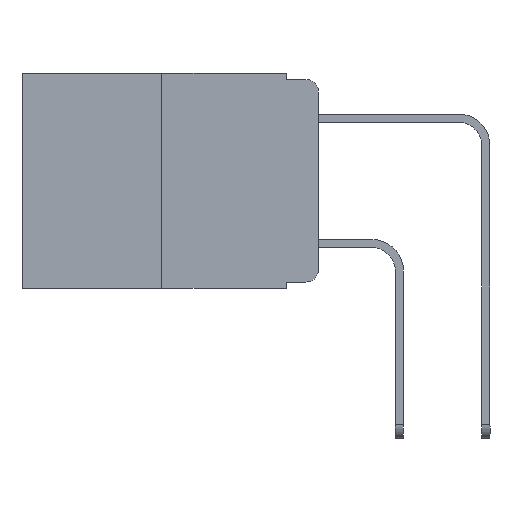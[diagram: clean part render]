
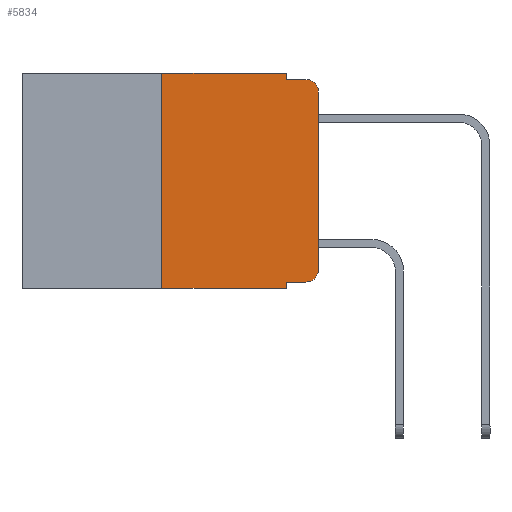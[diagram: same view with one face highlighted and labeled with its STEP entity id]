
A CAD part, left-side view. The second image highlights one B-rep face of the part: STEP entity #5834.
In plain terms, the highlighted planar face has unit normal (-1, 0, 0).
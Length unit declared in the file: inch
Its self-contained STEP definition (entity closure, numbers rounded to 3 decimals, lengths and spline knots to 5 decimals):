
#382 = CARTESIAN_POINT ( 'NONE',  ( 0., 0.051, -0.333 ) ) ;
#771 = CARTESIAN_POINT ( 'NONE',  ( 0., 0.25, 0. ) ) ;
#827 = CARTESIAN_POINT ( 'NONE',  ( 0., 0.473, 0. ) ) ;
#883 = CARTESIAN_POINT ( 'NONE',  ( 0., 0., 0. ) ) ;
#1315 = EDGE_CURVE ( 'NONE', #7490, #17654, #11008, .T. ) ;
#1879 = CARTESIAN_POINT ( 'NONE',  ( 0., 0.051, -0.343 ) ) ;
#2138 = DIRECTION ( 'NONE',  ( 0., 0., 1. ) ) ;
#2146 = DIRECTION ( 'NONE',  ( -1., 0., 0. ) ) ;
#2339 = CARTESIAN_POINT ( 'NONE',  ( 0., 0.051, 0. ) ) ;
#2368 = DIRECTION ( 'NONE',  ( -1., 0., 0. ) ) ;
#2535 = DIRECTION ( 'NONE',  ( 0., -1., 0. ) ) ;
#2853 = EDGE_CURVE ( 'NONE', #7490, #3936, #18631, .T. ) ;
#3482 = EDGE_CURVE ( 'NONE', #6286, #12022, #12248, .T. ) ;
#3511 = ORIENTED_EDGE ( 'NONE', *, *, #8426, .F. ) ;
#3579 = ORIENTED_EDGE ( 'NONE', *, *, #7062, .F. ) ;
#3762 = LINE ( 'NONE', #17247, #12461 ) ;
#3936 = VERTEX_POINT ( 'NONE', #6505 ) ;
#3972 = ORIENTED_EDGE ( 'NONE', *, *, #3482, .T. ) ;
#4372 = AXIS2_PLACEMENT_3D ( 'NONE', #827, #8157, #5220 ) ;
#4924 = EDGE_CURVE ( 'NONE', #9621, #9462, #5267, .T. ) ;
#5220 = DIRECTION ( 'NONE',  ( 0., 0., -1. ) ) ;
#5251 = DIRECTION ( 'NONE',  ( 0., 0., -1. ) ) ;
#5267 = LINE ( 'NONE', #5469, #11663 ) ;
#5469 = CARTESIAN_POINT ( 'NONE',  ( 0., 0.051, -0.01 ) ) ;
#5834 = ADVANCED_FACE ( 'NONE', ( #9622 ), #12666, .F. ) ;
#5928 = VECTOR ( 'NONE', #12631, 39.37008 ) ;
#6145 = EDGE_CURVE ( 'NONE', #11468, #17654, #9012, .T. ) ;
#6286 = VERTEX_POINT ( 'NONE', #15931 ) ;
#6471 = EDGE_CURVE ( 'NONE', #11468, #6286, #16497, .T. ) ;
#6501 = CARTESIAN_POINT ( 'NONE',  ( 0., 0., -0.313 ) ) ;
#6505 = CARTESIAN_POINT ( 'NONE',  ( 0., 0.25, 0. ) ) ;
#6548 = LINE ( 'NONE', #883, #5928 ) ;
#6814 = CARTESIAN_POINT ( 'NONE',  ( 0., 0.02, -0.313 ) ) ;
#7062 = EDGE_CURVE ( 'NONE', #3936, #18448, #3762, .T. ) ;
#7082 = CARTESIAN_POINT ( 'NONE',  ( 0., 0., -0.03 ) ) ;
#7239 = AXIS2_PLACEMENT_3D ( 'NONE', #6814, #2146, #15828 ) ;
#7403 = CARTESIAN_POINT ( 'NONE',  ( 0., 0.051, -0.333 ) ) ;
#7490 = VERTEX_POINT ( 'NONE', #18488 ) ;
#7547 = CARTESIAN_POINT ( 'NONE',  ( 0., 0.051, 0. ) ) ;
#8157 = DIRECTION ( 'NONE',  ( 1., 0., 0. ) ) ;
#8247 = VECTOR ( 'NONE', #2138, 39.37008 ) ;
#8426 = EDGE_CURVE ( 'NONE', #18448, #9621, #14250, .T. ) ;
#8751 = CIRCLE ( 'NONE', #15941, 0.02 ) ;
#9012 = LINE ( 'NONE', #7547, #10010 ) ;
#9462 = VERTEX_POINT ( 'NONE', #17594 ) ;
#9621 = VERTEX_POINT ( 'NONE', #18266 ) ;
#9622 = FACE_OUTER_BOUND ( 'NONE', #18646, .T. ) ;
#10010 = VECTOR ( 'NONE', #10596, 39.37008 ) ;
#10173 = ORIENTED_EDGE ( 'NONE', *, *, #6471, .T. ) ;
#10193 = ORIENTED_EDGE ( 'NONE', *, *, #4924, .F. ) ;
#10444 = CARTESIAN_POINT ( 'NONE',  ( 0., 0.051, 0. ) ) ;
#10596 = DIRECTION ( 'NONE',  ( 0., 0., -1. ) ) ;
#10724 = VECTOR ( 'NONE', #12445, 39.37008 ) ;
#10856 = DIRECTION ( 'NONE',  ( 0., -1., 0. ) ) ;
#11008 = LINE ( 'NONE', #11185, #10724 ) ;
#11115 = DIRECTION ( 'NONE',  ( 0., -1., 0. ) ) ;
#11185 = CARTESIAN_POINT ( 'NONE',  ( 0., 0.473, -0.343 ) ) ;
#11468 = VERTEX_POINT ( 'NONE', #7403 ) ;
#11663 = VECTOR ( 'NONE', #2535, 39.37008 ) ;
#12022 = VERTEX_POINT ( 'NONE', #6501 ) ;
#12248 = CIRCLE ( 'NONE', #7239, 0.02 ) ;
#12445 = DIRECTION ( 'NONE',  ( 0., -1., 0. ) ) ;
#12461 = VECTOR ( 'NONE', #11115, 39.37008 ) ;
#12631 = DIRECTION ( 'NONE',  ( 0., 0., 1. ) ) ;
#12666 = PLANE ( 'NONE',  #4372 ) ;
#13814 = VECTOR ( 'NONE', #5251, 39.37008 ) ;
#13868 = ORIENTED_EDGE ( 'NONE', *, *, #17734, .T. ) ;
#13875 = ORIENTED_EDGE ( 'NONE', *, *, #1315, .T. ) ;
#13994 = DIRECTION ( 'NONE',  ( 0., 0., -1. ) ) ;
#14250 = LINE ( 'NONE', #2339, #13814 ) ;
#14373 = CARTESIAN_POINT ( 'NONE',  ( 0., 0.02, -0.03 ) ) ;
#15828 = DIRECTION ( 'NONE',  ( 0., 0., -1. ) ) ;
#15931 = CARTESIAN_POINT ( 'NONE',  ( 0., 0.02, -0.333 ) ) ;
#15941 = AXIS2_PLACEMENT_3D ( 'NONE', #14373, #2368, #13994 ) ;
#16497 = LINE ( 'NONE', #382, #18695 ) ;
#16993 = VERTEX_POINT ( 'NONE', #7082 ) ;
#17247 = CARTESIAN_POINT ( 'NONE',  ( 0., 0.473, 0. ) ) ;
#17594 = CARTESIAN_POINT ( 'NONE',  ( 0., 0.02, -0.01 ) ) ;
#17654 = VERTEX_POINT ( 'NONE', #1879 ) ;
#17734 = EDGE_CURVE ( 'NONE', #16993, #9462, #8751, .T. ) ;
#17797 = EDGE_CURVE ( 'NONE', #12022, #16993, #6548, .T. ) ;
#18266 = CARTESIAN_POINT ( 'NONE',  ( 0., 0.051, -0.01 ) ) ;
#18378 = ORIENTED_EDGE ( 'NONE', *, *, #2853, .F. ) ;
#18448 = VERTEX_POINT ( 'NONE', #10444 ) ;
#18488 = CARTESIAN_POINT ( 'NONE',  ( 0., 0.25, -0.343 ) ) ;
#18571 = ORIENTED_EDGE ( 'NONE', *, *, #6145, .F. ) ;
#18631 = LINE ( 'NONE', #771, #8247 ) ;
#18646 = EDGE_LOOP ( 'NONE', ( #18963, #13868, #10193, #3511, #3579, #18378, #13875, #18571, #10173, #3972 ) ) ;
#18695 = VECTOR ( 'NONE', #10856, 39.37008 ) ;
#18963 = ORIENTED_EDGE ( 'NONE', *, *, #17797, .T. ) ;
